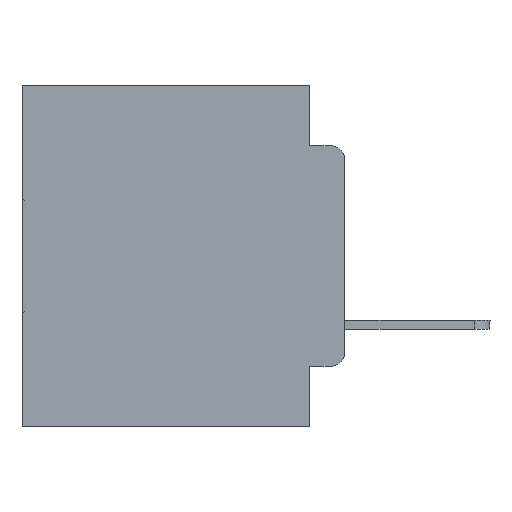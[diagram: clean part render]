
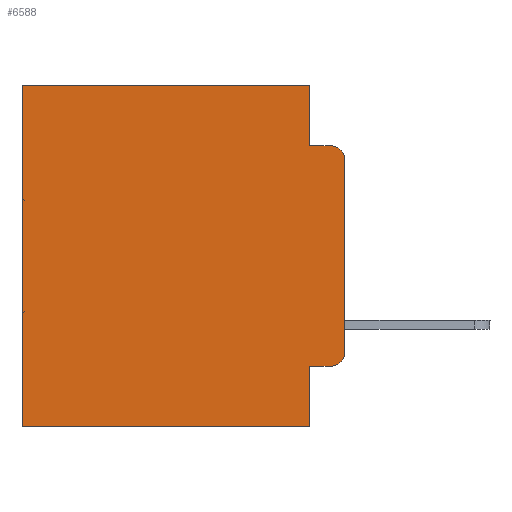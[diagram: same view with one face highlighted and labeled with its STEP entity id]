
A CAD part, left-side view. The second image highlights one B-rep face of the part: STEP entity #6588.
In plain terms, the highlighted planar face has unit normal (-1, 0, 0).
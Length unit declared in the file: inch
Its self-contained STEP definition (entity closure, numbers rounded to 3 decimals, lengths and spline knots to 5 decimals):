
#126 = VECTOR ( 'NONE', #14907, 39.37008 ) ;
#152 = VECTOR ( 'NONE', #24315, 39.37008 ) ;
#426 = LINE ( 'NONE', #3428, #31768 ) ;
#593 = EDGE_CURVE ( 'NONE', #20901, #20510, #29199, .T. ) ;
#1199 = CARTESIAN_POINT ( 'NONE',  ( 0.298, 0.473, 0. ) ) ;
#2715 = EDGE_LOOP ( 'NONE', ( #8417, #25214, #16839, #5584, #24295, #22482, #31160, #14350, #12709, #27854 ) ) ;
#2854 = DIRECTION ( 'NONE',  ( 0., 0., -1. ) ) ;
#3310 = EDGE_CURVE ( 'NONE', #12492, #5915, #9433, .T. ) ;
#3313 = CARTESIAN_POINT ( 'NONE',  ( 0.298, 0.02, -0.3915 ) ) ;
#3428 = CARTESIAN_POINT ( 'NONE',  ( 0.298, 0., 0. ) ) ;
#3822 = CARTESIAN_POINT ( 'NONE',  ( 0.298, 0.051, 0. ) ) ;
#4347 = EDGE_CURVE ( 'NONE', #28554, #18414, #12134, .T. ) ;
#5244 = LINE ( 'NONE', #1199, #28952 ) ;
#5383 = DIRECTION ( 'NONE',  ( 1., 0., 0. ) ) ;
#5584 = ORIENTED_EDGE ( 'NONE', *, *, #25370, .F. ) ;
#5915 = VERTEX_POINT ( 'NONE', #5928 ) ;
#5928 = CARTESIAN_POINT ( 'NONE',  ( 0.298, 0.473, -0.5 ) ) ;
#6110 = VECTOR ( 'NONE', #26452, 39.37008 ) ;
#6563 = AXIS2_PLACEMENT_3D ( 'NONE', #20494, #27607, #2854 ) ;
#6588 = ADVANCED_FACE ( 'NONE', ( #12744 ), #18168, .F. ) ;
#6964 = LINE ( 'NONE', #15106, #126 ) ;
#8417 = ORIENTED_EDGE ( 'NONE', *, *, #11382, .F. ) ;
#8950 = AXIS2_PLACEMENT_3D ( 'NONE', #3313, #22819, #20647 ) ;
#9433 = LINE ( 'NONE', #31337, #25378 ) ;
#10596 = VECTOR ( 'NONE', #25472, 39.37008 ) ;
#11359 = VECTOR ( 'NONE', #22987, 39.37008 ) ;
#11382 = EDGE_CURVE ( 'NONE', #27933, #31903, #426, .T. ) ;
#11923 = CARTESIAN_POINT ( 'NONE',  ( 0.298, 0.473, 0. ) ) ;
#12020 = CARTESIAN_POINT ( 'NONE',  ( 0.298, 0., 0. ) ) ;
#12112 = DIRECTION ( 'NONE',  ( 0., 1., 0. ) ) ;
#12134 = LINE ( 'NONE', #30632, #11359 ) ;
#12492 = VERTEX_POINT ( 'NONE', #13865 ) ;
#12701 = AXIS2_PLACEMENT_3D ( 'NONE', #30618, #5383, #20692 ) ;
#12709 = ORIENTED_EDGE ( 'NONE', *, *, #4347, .T. ) ;
#12744 = FACE_OUTER_BOUND ( 'NONE', #2715, .T. ) ;
#12966 = CARTESIAN_POINT ( 'NONE',  ( 0.298, 0., -0.3915 ) ) ;
#13865 = CARTESIAN_POINT ( 'NONE',  ( 0.298, 0.051, -0.5 ) ) ;
#13971 = CIRCLE ( 'NONE', #8950, 0.02 ) ;
#14350 = ORIENTED_EDGE ( 'NONE', *, *, #31811, .F. ) ;
#14907 = DIRECTION ( 'NONE',  ( 0., -1., 0. ) ) ;
#15106 = CARTESIAN_POINT ( 'NONE',  ( 0.298, 0.051, -0.0885 ) ) ;
#15519 = DIRECTION ( 'NONE',  ( 0., 0., -1. ) ) ;
#15587 = CARTESIAN_POINT ( 'NONE',  ( 0.298, 0.051, 0. ) ) ;
#16355 = EDGE_CURVE ( 'NONE', #18414, #31903, #13971, .T. ) ;
#16839 = ORIENTED_EDGE ( 'NONE', *, *, #24059, .F. ) ;
#17582 = CARTESIAN_POINT ( 'NONE',  ( 0.298, 0.02, -0.0885 ) ) ;
#18168 = PLANE ( 'NONE',  #12701 ) ;
#18414 = VERTEX_POINT ( 'NONE', #22934 ) ;
#20494 = CARTESIAN_POINT ( 'NONE',  ( 0.298, 0.02, -0.1085 ) ) ;
#20510 = VERTEX_POINT ( 'NONE', #11923 ) ;
#20647 = DIRECTION ( 'NONE',  ( 0., 0., -1. ) ) ;
#20692 = DIRECTION ( 'NONE',  ( 0., 0., -1. ) ) ;
#20901 = VERTEX_POINT ( 'NONE', #21279 ) ;
#21279 = CARTESIAN_POINT ( 'NONE',  ( 0.298, 0.051, 0. ) ) ;
#21374 = EDGE_CURVE ( 'NONE', #20510, #5915, #5244, .T. ) ;
#21902 = CARTESIAN_POINT ( 'NONE',  ( 0.298, 0.051, -0.0885 ) ) ;
#21935 = CIRCLE ( 'NONE', #6563, 0.02 ) ;
#22482 = ORIENTED_EDGE ( 'NONE', *, *, #21374, .T. ) ;
#22819 = DIRECTION ( 'NONE',  ( -1., 0., 0. ) ) ;
#22934 = CARTESIAN_POINT ( 'NONE',  ( 0.298, 0.02, -0.4115 ) ) ;
#22987 = DIRECTION ( 'NONE',  ( 0., -1., 0. ) ) ;
#24059 = EDGE_CURVE ( 'NONE', #29885, #24843, #6964, .T. ) ;
#24295 = ORIENTED_EDGE ( 'NONE', *, *, #593, .T. ) ;
#24315 = DIRECTION ( 'NONE',  ( 0., 1., 0. ) ) ;
#24843 = VERTEX_POINT ( 'NONE', #17582 ) ;
#25214 = ORIENTED_EDGE ( 'NONE', *, *, #31883, .T. ) ;
#25370 = EDGE_CURVE ( 'NONE', #20901, #29885, #31370, .T. ) ;
#25378 = VECTOR ( 'NONE', #12112, 39.37008 ) ;
#25472 = DIRECTION ( 'NONE',  ( 0., 0., -1. ) ) ;
#26452 = DIRECTION ( 'NONE',  ( 0., 0., -1. ) ) ;
#27607 = DIRECTION ( 'NONE',  ( -1., 0., 0. ) ) ;
#27854 = ORIENTED_EDGE ( 'NONE', *, *, #16355, .T. ) ;
#27933 = VERTEX_POINT ( 'NONE', #31614 ) ;
#28499 = LINE ( 'NONE', #15587, #10596 ) ;
#28554 = VERTEX_POINT ( 'NONE', #31816 ) ;
#28952 = VECTOR ( 'NONE', #30804, 39.37008 ) ;
#29199 = LINE ( 'NONE', #12020, #152 ) ;
#29885 = VERTEX_POINT ( 'NONE', #21902 ) ;
#30618 = CARTESIAN_POINT ( 'NONE',  ( 0.298, 0., 0. ) ) ;
#30632 = CARTESIAN_POINT ( 'NONE',  ( 0.298, 0.051, -0.4115 ) ) ;
#30804 = DIRECTION ( 'NONE',  ( 0., 0., -1. ) ) ;
#31160 = ORIENTED_EDGE ( 'NONE', *, *, #3310, .F. ) ;
#31337 = CARTESIAN_POINT ( 'NONE',  ( 0.298, 0., -0.5 ) ) ;
#31370 = LINE ( 'NONE', #3822, #6110 ) ;
#31614 = CARTESIAN_POINT ( 'NONE',  ( 0.298, 0., -0.1085 ) ) ;
#31768 = VECTOR ( 'NONE', #15519, 39.37008 ) ;
#31811 = EDGE_CURVE ( 'NONE', #28554, #12492, #28499, .T. ) ;
#31816 = CARTESIAN_POINT ( 'NONE',  ( 0.298, 0.051, -0.4115 ) ) ;
#31883 = EDGE_CURVE ( 'NONE', #27933, #24843, #21935, .T. ) ;
#31903 = VERTEX_POINT ( 'NONE', #12966 ) ;
